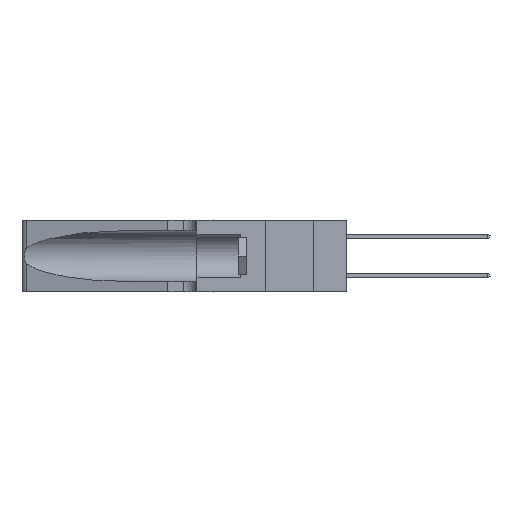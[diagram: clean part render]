
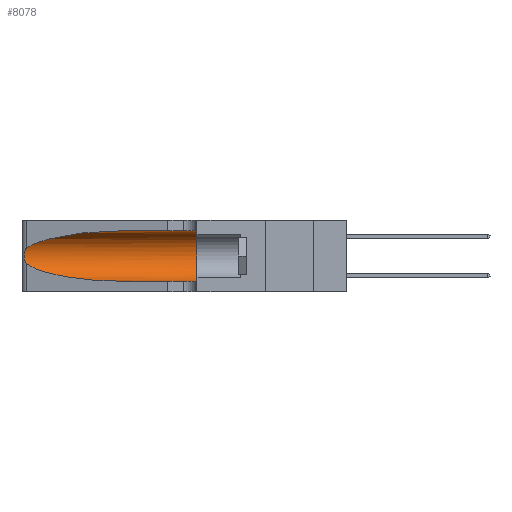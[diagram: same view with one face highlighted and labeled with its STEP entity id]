
A CAD part, left-side view. The second image highlights one B-rep face of the part: STEP entity #8078.
In plain terms, the highlighted cylindrical face has radius 3.308 mm (diameter 6.617 mm), a partial arc.
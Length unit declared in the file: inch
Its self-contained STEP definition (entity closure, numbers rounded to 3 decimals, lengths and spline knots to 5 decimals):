
#304 = DIRECTION ( 'NONE',  ( 0., -1., 0. ) ) ;
#1392 = CARTESIAN_POINT ( 'NONE',  ( 0.25555, 1.22994, 0.2215 ) ) ;
#2359 =( BOUNDED_CURVE ( )  B_SPLINE_CURVE ( 3, ( #14977, #3973, #8244, #23167 ),
 .UNSPECIFIED., .F., .T. ) 
 B_SPLINE_CURVE_WITH_KNOTS ( ( 4, 4 ),
 ( 1.5708, 2.84003 ),
 .UNSPECIFIED. ) 
 CURVE ( )  GEOMETRIC_REPRESENTATION_ITEM ( )  RATIONAL_B_SPLINE_CURVE ( ( 1., 0.87, 0.87, 1. ) ) 
 REPRESENTATION_ITEM ( '' )  );
#3186 = CYLINDRICAL_SURFACE ( 'NONE', #9664, 0.13025 ) ;
#3973 = CARTESIAN_POINT ( 'NONE',  ( 0.18966, 0.96281, 0.31525 ) ) ;
#4535 = ORIENTED_EDGE ( 'NONE', *, *, #20203, .T. ) ;
#4720 = B_SPLINE_CURVE_WITH_KNOTS ( 'NONE', 3,
 ( #9922, #1392, #27208, #18597, #25083, #26937, #7751, #22701, #14224, #7839, #12080, #12270, #14519, #27028 ),
 .UNSPECIFIED., .F., .F.,
 ( 4, 2, 2, 2, 2, 2, 4 ),
 ( 0., 0.00027, 0.00053, 0.00107, 0.0016, 0.00187, 0.00214 ),
 .UNSPECIFIED. ) ;
#4977 = CIRCLE ( 'NONE', #9872, 0.13025 ) ;
#5471 = VERTEX_POINT ( 'NONE', #25378 ) ;
#5742 = DIRECTION ( 'NONE',  ( 0., -1., 0. ) ) ;
#5838 = FACE_OUTER_BOUND ( 'NONE', #17017, .T. ) ;
#6460 = VECTOR ( 'NONE', #8057, 39.37008 ) ;
#6903 = VERTEX_POINT ( 'NONE', #22845 ) ;
#7239 = ORIENTED_EDGE ( 'NONE', *, *, #17240, .T. ) ;
#7751 = CARTESIAN_POINT ( 'NONE',  ( 0.26075, 1.23896, 0.19203 ) ) ;
#7839 = CARTESIAN_POINT ( 'NONE',  ( 0.25856, 1.23593, 0.16098 ) ) ;
#7907 = VERTEX_POINT ( 'NONE', #9567 ) ;
#7986 = ORIENTED_EDGE ( 'NONE', *, *, #8288, .F. ) ;
#8057 = DIRECTION ( 'NONE',  ( 0., -1., 0. ) ) ;
#8078 = ADVANCED_FACE ( 'NONE', ( #5838 ), #3186, .F. ) ;
#8244 = CARTESIAN_POINT ( 'NONE',  ( 0.2373, 1.15595, 0.28018 ) ) ;
#8288 = EDGE_CURVE ( 'NONE', #9359, #19400, #13848, .T. ) ;
#9359 = VERTEX_POINT ( 'NONE', #9669 ) ;
#9567 = CARTESIAN_POINT ( 'NONE',  ( 0.1305, 0.72297, 0.05475 ) ) ;
#9664 = AXIS2_PLACEMENT_3D ( 'NONE', #18451, #5742, #12836 ) ;
#9669 = CARTESIAN_POINT ( 'NONE',  ( 0.1305, 0.72297, 0.31525 ) ) ;
#9872 = AXIS2_PLACEMENT_3D ( 'NONE', #11100, #24019, #11015 ) ;
#9922 = CARTESIAN_POINT ( 'NONE',  ( 0.25487, 1.22718, 0.22369 ) ) ;
#10855 = VERTEX_POINT ( 'NONE', #20941 ) ;
#11015 = DIRECTION ( 'NONE',  ( 0., 0., 1. ) ) ;
#11100 = CARTESIAN_POINT ( 'NONE',  ( 0.1305, 0.35, 0.185 ) ) ;
#12080 = CARTESIAN_POINT ( 'NONE',  ( 0.25789, 1.23486, 0.15765 ) ) ;
#12270 = CARTESIAN_POINT ( 'NONE',  ( 0.25639, 1.23186, 0.15144 ) ) ;
#12483 = VECTOR ( 'NONE', #304, 39.37008 ) ;
#12836 = DIRECTION ( 'NONE',  ( 0., 0., -1. ) ) ;
#13132 =( BOUNDED_CURVE ( )  B_SPLINE_CURVE ( 3, ( #15164, #25651, #15256, #17379 ),
 .UNSPECIFIED., .F., .F. ) 
 B_SPLINE_CURVE_WITH_KNOTS ( ( 4, 4 ),
 ( 3.44316, 4.71239 ),
 .UNSPECIFIED. ) 
 CURVE ( )  GEOMETRIC_REPRESENTATION_ITEM ( )  RATIONAL_B_SPLINE_CURVE ( ( 1., 0.87, 0.87, 1. ) ) 
 REPRESENTATION_ITEM ( '' )  );
#13820 = ORIENTED_EDGE ( 'NONE', *, *, #20136, .F. ) ;
#13848 = LINE ( 'NONE', #23888, #6460 ) ;
#14224 = CARTESIAN_POINT ( 'NONE',  ( 0.26017, 1.23833, 0.17102 ) ) ;
#14519 = CARTESIAN_POINT ( 'NONE',  ( 0.25555, 1.22993, 0.14849 ) ) ;
#14977 = CARTESIAN_POINT ( 'NONE',  ( 0.1305, 0.72297, 0.31525 ) ) ;
#15148 = LINE ( 'NONE', #18929, #12483 ) ;
#15164 = CARTESIAN_POINT ( 'NONE',  ( 0.25487, 1.22718, 0.14631 ) ) ;
#15256 = CARTESIAN_POINT ( 'NONE',  ( 0.18966, 0.96281, 0.05475 ) ) ;
#15535 = CARTESIAN_POINT ( 'NONE',  ( 0.1305, 0.35, 0.31525 ) ) ;
#17017 = EDGE_LOOP ( 'NONE', ( #18236, #26366, #7239, #4535, #13820, #7986 ) ) ;
#17240 = EDGE_CURVE ( 'NONE', #5471, #7907, #13132, .T. ) ;
#17379 = CARTESIAN_POINT ( 'NONE',  ( 0.1305, 0.72297, 0.05475 ) ) ;
#18236 = ORIENTED_EDGE ( 'NONE', *, *, #24841, .T. ) ;
#18451 = CARTESIAN_POINT ( 'NONE',  ( 0.1305, 1.61858, 0.185 ) ) ;
#18597 = CARTESIAN_POINT ( 'NONE',  ( 0.25787, 1.23484, 0.2124 ) ) ;
#18929 = CARTESIAN_POINT ( 'NONE',  ( 0.1305, 1.61858, 0.05475 ) ) ;
#19269 = EDGE_CURVE ( 'NONE', #10855, #5471, #4720, .T. ) ;
#19400 = VERTEX_POINT ( 'NONE', #15535 ) ;
#20136 = EDGE_CURVE ( 'NONE', #19400, #6903, #4977, .T. ) ;
#20203 = EDGE_CURVE ( 'NONE', #7907, #6903, #15148, .T. ) ;
#20941 = CARTESIAN_POINT ( 'NONE',  ( 0.25487, 1.22718, 0.22369 ) ) ;
#22701 = CARTESIAN_POINT ( 'NONE',  ( 0.26075, 1.23896, 0.178 ) ) ;
#22845 = CARTESIAN_POINT ( 'NONE',  ( 0.1305, 0.35, 0.05475 ) ) ;
#23167 = CARTESIAN_POINT ( 'NONE',  ( 0.25487, 1.22718, 0.22369 ) ) ;
#23888 = CARTESIAN_POINT ( 'NONE',  ( 0.1305, 1.61858, 0.31525 ) ) ;
#24019 = DIRECTION ( 'NONE',  ( 0., 1., 0. ) ) ;
#24841 = EDGE_CURVE ( 'NONE', #9359, #10855, #2359, .T. ) ;
#25083 = CARTESIAN_POINT ( 'NONE',  ( 0.25854, 1.2359, 0.20912 ) ) ;
#25378 = CARTESIAN_POINT ( 'NONE',  ( 0.25487, 1.22718, 0.14631 ) ) ;
#25651 = CARTESIAN_POINT ( 'NONE',  ( 0.2373, 1.15595, 0.08982 ) ) ;
#26366 = ORIENTED_EDGE ( 'NONE', *, *, #19269, .T. ) ;
#26937 = CARTESIAN_POINT ( 'NONE',  ( 0.26018, 1.23835, 0.19895 ) ) ;
#27028 = CARTESIAN_POINT ( 'NONE',  ( 0.25487, 1.22718, 0.14631 ) ) ;
#27208 = CARTESIAN_POINT ( 'NONE',  ( 0.25639, 1.23184, 0.21858 ) ) ;
